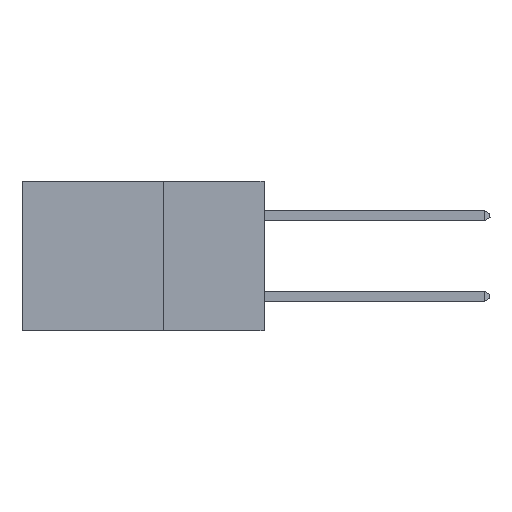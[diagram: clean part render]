
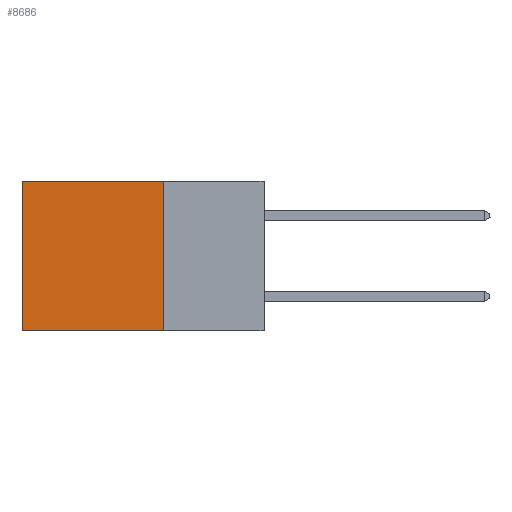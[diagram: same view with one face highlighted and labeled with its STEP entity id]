
A CAD part, left-side view. The second image highlights one B-rep face of the part: STEP entity #8686.
In plain terms, the highlighted planar face has unit normal (-1, 0, 0).
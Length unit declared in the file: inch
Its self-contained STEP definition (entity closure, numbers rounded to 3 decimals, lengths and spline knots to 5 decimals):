
#36 = CARTESIAN_POINT ( 'NONE',  ( 0.298, 0.25, 0. ) ) ;
#864 = VECTOR ( 'NONE', #3443, 39.37008 ) ;
#928 = VECTOR ( 'NONE', #9010, 39.37008 ) ;
#1172 = ORIENTED_EDGE ( 'NONE', *, *, #8645, .T. ) ;
#1335 = DIRECTION ( 'NONE',  ( 0., 0., -1. ) ) ;
#1429 = CARTESIAN_POINT ( 'NONE',  ( 0.298, 0.6, 0. ) ) ;
#1757 = VERTEX_POINT ( 'NONE', #7537 ) ;
#2265 = VERTEX_POINT ( 'NONE', #5299 ) ;
#2912 = AXIS2_PLACEMENT_3D ( 'NONE', #4879, #8198, #6521 ) ;
#3270 = FACE_OUTER_BOUND ( 'NONE', #9249, .T. ) ;
#3427 = ORIENTED_EDGE ( 'NONE', *, *, #5107, .F. ) ;
#3443 = DIRECTION ( 'NONE',  ( 0., 1., 0. ) ) ;
#3469 = ORIENTED_EDGE ( 'NONE', *, *, #4986, .F. ) ;
#3931 = LINE ( 'NONE', #1429, #9580 ) ;
#4121 = CARTESIAN_POINT ( 'NONE',  ( 0.298, 0.25, 0. ) ) ;
#4231 = ORIENTED_EDGE ( 'NONE', *, *, #8850, .T. ) ;
#4698 = LINE ( 'NONE', #36, #864 ) ;
#4777 = PLANE ( 'NONE',  #2912 ) ;
#4879 = CARTESIAN_POINT ( 'NONE',  ( 0.298, 0.25, 0. ) ) ;
#4986 = EDGE_CURVE ( 'NONE', #2265, #9102, #5026, .T. ) ;
#5026 = LINE ( 'NONE', #7067, #6979 ) ;
#5107 = EDGE_CURVE ( 'NONE', #1757, #2265, #10182, .T. ) ;
#5299 = CARTESIAN_POINT ( 'NONE',  ( 0.298, 0.25, -0.37 ) ) ;
#6521 = DIRECTION ( 'NONE',  ( 0., 0., -1. ) ) ;
#6979 = VECTOR ( 'NONE', #8748, 39.37008 ) ;
#7067 = CARTESIAN_POINT ( 'NONE',  ( 0.298, 0.25, -0.37 ) ) ;
#7537 = CARTESIAN_POINT ( 'NONE',  ( 0.298, 0.25, 0. ) ) ;
#8198 = DIRECTION ( 'NONE',  ( 1., 0., 0. ) ) ;
#8645 = EDGE_CURVE ( 'NONE', #8858, #9102, #3931, .T. ) ;
#8682 = CARTESIAN_POINT ( 'NONE',  ( 0.298, 0.6, -0.37 ) ) ;
#8686 = ADVANCED_FACE ( 'NONE', ( #3270 ), #4777, .F. ) ;
#8748 = DIRECTION ( 'NONE',  ( 0., 1., 0. ) ) ;
#8850 = EDGE_CURVE ( 'NONE', #1757, #8858, #4698, .T. ) ;
#8858 = VERTEX_POINT ( 'NONE', #9145 ) ;
#9010 = DIRECTION ( 'NONE',  ( 0., 0., -1. ) ) ;
#9102 = VERTEX_POINT ( 'NONE', #8682 ) ;
#9145 = CARTESIAN_POINT ( 'NONE',  ( 0.298, 0.6, 0. ) ) ;
#9249 = EDGE_LOOP ( 'NONE', ( #1172, #3469, #3427, #4231 ) ) ;
#9580 = VECTOR ( 'NONE', #1335, 39.37008 ) ;
#10182 = LINE ( 'NONE', #4121, #928 ) ;
